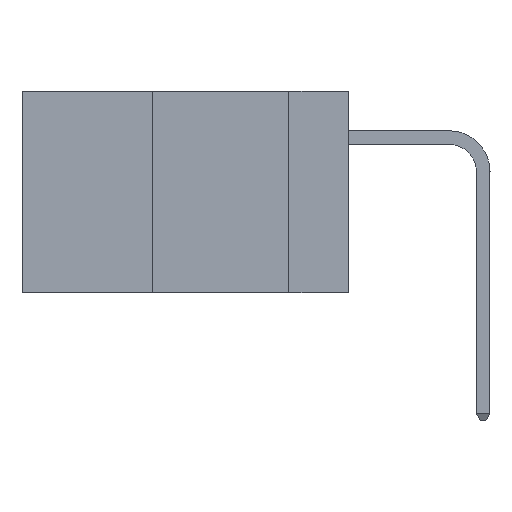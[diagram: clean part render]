
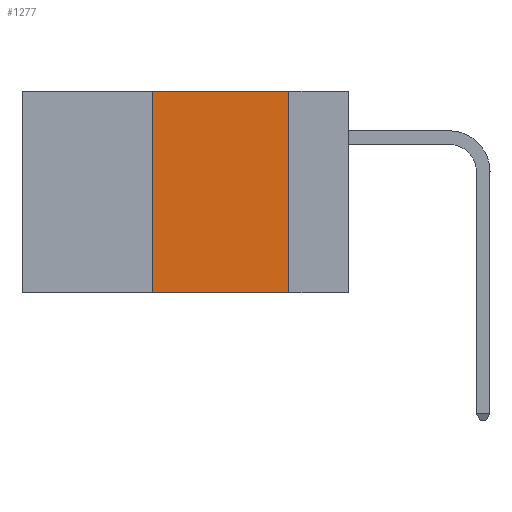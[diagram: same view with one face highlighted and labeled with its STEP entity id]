
A CAD part, left-side view. The second image highlights one B-rep face of the part: STEP entity #1277.
In plain terms, the highlighted planar face has unit normal (-1, 0, 0).
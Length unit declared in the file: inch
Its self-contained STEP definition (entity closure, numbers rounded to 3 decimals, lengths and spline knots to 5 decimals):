
#1277 = ADVANCED_FACE ( 'NONE', ( #13068 ), #14972, .F. ) ;
#1633 = ORIENTED_EDGE ( 'NONE', *, *, #4153, .F. ) ;
#1763 = EDGE_CURVE ( 'NONE', #4802, #17887, #11432, .T. ) ;
#2163 = CARTESIAN_POINT ( 'NONE',  ( 0., 0.11, -0.37 ) ) ;
#4153 = EDGE_CURVE ( 'NONE', #4802, #8660, #21054, .T. ) ;
#4623 = VECTOR ( 'NONE', #9852, 39.37008 ) ;
#4802 = VERTEX_POINT ( 'NONE', #11118 ) ;
#6863 = ORIENTED_EDGE ( 'NONE', *, *, #1763, .T. ) ;
#7876 = DIRECTION ( 'NONE',  ( 0., -1., 0. ) ) ;
#8660 = VERTEX_POINT ( 'NONE', #17484 ) ;
#8691 = CARTESIAN_POINT ( 'NONE',  ( 0., 0.11, 0. ) ) ;
#9171 = ORIENTED_EDGE ( 'NONE', *, *, #9820, .F. ) ;
#9799 = CARTESIAN_POINT ( 'NONE',  ( 0., 0.6, 0. ) ) ;
#9820 = EDGE_CURVE ( 'NONE', #17334, #17887, #10483, .T. ) ;
#9852 = DIRECTION ( 'NONE',  ( 0., -1., 0. ) ) ;
#10483 = LINE ( 'NONE', #8691, #19470 ) ;
#10954 = EDGE_LOOP ( 'NONE', ( #9171, #19188, #1633, #6863 ) ) ;
#11118 = CARTESIAN_POINT ( 'NONE',  ( 0., 0.36, -0.37 ) ) ;
#11147 = CARTESIAN_POINT ( 'NONE',  ( 0., 0.36, 0. ) ) ;
#11234 = DIRECTION ( 'NONE',  ( 0., 0., -1. ) ) ;
#11432 = LINE ( 'NONE', #19578, #20377 ) ;
#11718 = AXIS2_PLACEMENT_3D ( 'NONE', #9799, #12337, #11234 ) ;
#12131 = VECTOR ( 'NONE', #12601, 39.37008 ) ;
#12337 = DIRECTION ( 'NONE',  ( 1., 0., 0. ) ) ;
#12601 = DIRECTION ( 'NONE',  ( 0., 0., 1. ) ) ;
#13068 = FACE_OUTER_BOUND ( 'NONE', #10954, .T. ) ;
#14093 = CARTESIAN_POINT ( 'NONE',  ( 0., 0.11, 0. ) ) ;
#14972 = PLANE ( 'NONE',  #11718 ) ;
#16578 = CARTESIAN_POINT ( 'NONE',  ( 0., 0.6, 0. ) ) ;
#17334 = VERTEX_POINT ( 'NONE', #14093 ) ;
#17484 = CARTESIAN_POINT ( 'NONE',  ( 0., 0.36, 0. ) ) ;
#17887 = VERTEX_POINT ( 'NONE', #2163 ) ;
#18735 = DIRECTION ( 'NONE',  ( 0., 0., -1. ) ) ;
#19107 = LINE ( 'NONE', #16578, #4623 ) ;
#19188 = ORIENTED_EDGE ( 'NONE', *, *, #21256, .F. ) ;
#19470 = VECTOR ( 'NONE', #18735, 39.37008 ) ;
#19578 = CARTESIAN_POINT ( 'NONE',  ( 0., 0.6, -0.37 ) ) ;
#20377 = VECTOR ( 'NONE', #7876, 39.37008 ) ;
#21054 = LINE ( 'NONE', #11147, #12131 ) ;
#21256 = EDGE_CURVE ( 'NONE', #8660, #17334, #19107, .T. ) ;
